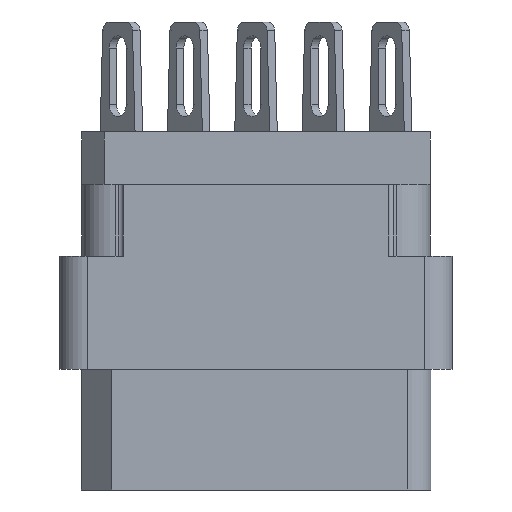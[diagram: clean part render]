
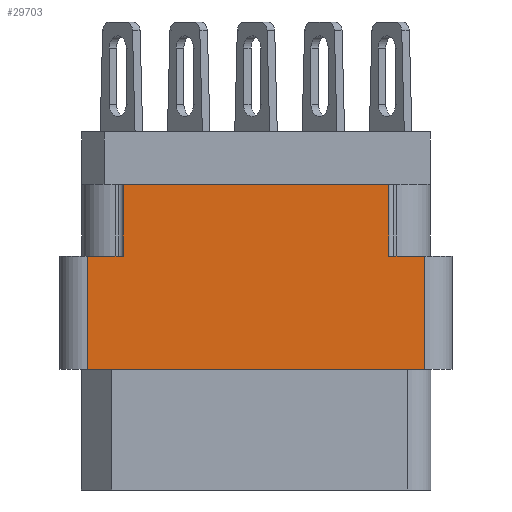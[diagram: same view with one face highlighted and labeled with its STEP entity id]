
A CAD part, left-side view. The second image highlights one B-rep face of the part: STEP entity #29703.
In plain terms, the highlighted planar face has unit normal (-1, 0, 0).
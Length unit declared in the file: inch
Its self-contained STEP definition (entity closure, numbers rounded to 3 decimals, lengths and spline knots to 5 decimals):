
#116 = CARTESIAN_POINT ( 'NONE',  ( -1., -0.376, -0.529 ) ) ;
#2129 = CARTESIAN_POINT ( 'NONE',  ( -1., -0.376, -0.529 ) ) ;
#2211 = LINE ( 'NONE', #35784, #32239 ) ;
#4123 = VECTOR ( 'NONE', #28141, 39.37008 ) ;
#4186 = ORIENTED_EDGE ( 'NONE', *, *, #26919, .F. ) ;
#4498 = DIRECTION ( 'NONE',  ( 0., -1., 0. ) ) ;
#4807 = DIRECTION ( 'NONE',  ( 0., -1., 0. ) ) ;
#5062 = CARTESIAN_POINT ( 'NONE',  ( -1., -0.296, -0.117 ) ) ;
#5085 = CARTESIAN_POINT ( 'NONE',  ( -1., -0.296, -0.277 ) ) ;
#5240 = LINE ( 'NONE', #19063, #13813 ) ;
#5653 = CARTESIAN_POINT ( 'NONE',  ( -1., 0.376, -0.798 ) ) ;
#5930 = VERTEX_POINT ( 'NONE', #9244 ) ;
#6096 = EDGE_CURVE ( 'NONE', #18663, #5930, #2211, .T. ) ;
#7786 = CARTESIAN_POINT ( 'NONE',  ( -1., 0.376, -0.529 ) ) ;
#9244 = CARTESIAN_POINT ( 'NONE',  ( -1., 0.296, -0.277 ) ) ;
#9344 = DIRECTION ( 'NONE',  ( -1., 0., 0. ) ) ;
#9796 = CARTESIAN_POINT ( 'NONE',  ( -1., -0.376, -0.277 ) ) ;
#10164 = VECTOR ( 'NONE', #32843, 39.37008 ) ;
#10178 = DIRECTION ( 'NONE',  ( 0., 0., 1. ) ) ;
#10691 = VERTEX_POINT ( 'NONE', #116 ) ;
#11288 = VECTOR ( 'NONE', #33193, 39.37008 ) ;
#11901 = EDGE_LOOP ( 'NONE', ( #26837, #4186, #26908, #22392, #35213, #28728, #31324, #19036 ) ) ;
#13813 = VECTOR ( 'NONE', #4498, 39.37008 ) ;
#13922 = DIRECTION ( 'NONE',  ( 0., 0., 1. ) ) ;
#14253 = VERTEX_POINT ( 'NONE', #9796 ) ;
#14954 = VERTEX_POINT ( 'NONE', #5062 ) ;
#15341 = EDGE_CURVE ( 'NONE', #10691, #14253, #30640, .T. ) ;
#15355 = VECTOR ( 'NONE', #18925, 39.37008 ) ;
#16679 = LINE ( 'NONE', #5085, #28107 ) ;
#18567 = FACE_OUTER_BOUND ( 'NONE', #11901, .T. ) ;
#18663 = VERTEX_POINT ( 'NONE', #21725 ) ;
#18925 = DIRECTION ( 'NONE',  ( 0., 1., 0. ) ) ;
#19036 = ORIENTED_EDGE ( 'NONE', *, *, #6096, .F. ) ;
#19063 = CARTESIAN_POINT ( 'NONE',  ( -1., 0.438, -0.117 ) ) ;
#19352 = VECTOR ( 'NONE', #10178, 39.37008 ) ;
#19531 = EDGE_CURVE ( 'NONE', #5930, #21313, #21591, .T. ) ;
#20542 = CARTESIAN_POINT ( 'NONE',  ( -1., -0.296, -0.277 ) ) ;
#21313 = VERTEX_POINT ( 'NONE', #34097 ) ;
#21591 = LINE ( 'NONE', #27662, #10164 ) ;
#21687 = LINE ( 'NONE', #2129, #15355 ) ;
#21725 = CARTESIAN_POINT ( 'NONE',  ( -1., 0.376, -0.277 ) ) ;
#22021 = AXIS2_PLACEMENT_3D ( 'NONE', #29068, #9344, #29811 ) ;
#22392 = ORIENTED_EDGE ( 'NONE', *, *, #25352, .F. ) ;
#24556 = CARTESIAN_POINT ( 'NONE',  ( -1., -0.376, -0.798 ) ) ;
#24701 = EDGE_CURVE ( 'NONE', #31984, #18663, #27955, .T. ) ;
#25352 = EDGE_CURVE ( 'NONE', #27173, #14253, #27096, .T. ) ;
#26837 = ORIENTED_EDGE ( 'NONE', *, *, #24701, .F. ) ;
#26908 = ORIENTED_EDGE ( 'NONE', *, *, #15341, .T. ) ;
#26919 = EDGE_CURVE ( 'NONE', #10691, #31984, #21687, .T. ) ;
#27096 = LINE ( 'NONE', #33383, #11288 ) ;
#27173 = VERTEX_POINT ( 'NONE', #20542 ) ;
#27662 = CARTESIAN_POINT ( 'NONE',  ( -1., 0.296, -0.277 ) ) ;
#27955 = LINE ( 'NONE', #5653, #4123 ) ;
#28107 = VECTOR ( 'NONE', #13922, 39.37008 ) ;
#28141 = DIRECTION ( 'NONE',  ( 0., 0., 1. ) ) ;
#28728 = ORIENTED_EDGE ( 'NONE', *, *, #30342, .F. ) ;
#29068 = CARTESIAN_POINT ( 'NONE',  ( -1., -0.376, -0.798 ) ) ;
#29703 = ADVANCED_FACE ( 'NONE', ( #18567 ), #34600, .T. ) ;
#29811 = DIRECTION ( 'NONE',  ( 0., 0., 1. ) ) ;
#30342 = EDGE_CURVE ( 'NONE', #21313, #14954, #5240, .T. ) ;
#30640 = LINE ( 'NONE', #24556, #19352 ) ;
#31324 = ORIENTED_EDGE ( 'NONE', *, *, #19531, .F. ) ;
#31984 = VERTEX_POINT ( 'NONE', #7786 ) ;
#32239 = VECTOR ( 'NONE', #4807, 39.37008 ) ;
#32843 = DIRECTION ( 'NONE',  ( 0., 0., 1. ) ) ;
#33193 = DIRECTION ( 'NONE',  ( 0., -1., 0. ) ) ;
#33383 = CARTESIAN_POINT ( 'NONE',  ( -1., -0.296, -0.277 ) ) ;
#33547 = EDGE_CURVE ( 'NONE', #27173, #14954, #16679, .T. ) ;
#34097 = CARTESIAN_POINT ( 'NONE',  ( -1., 0.296, -0.117 ) ) ;
#34600 = PLANE ( 'NONE',  #22021 ) ;
#35213 = ORIENTED_EDGE ( 'NONE', *, *, #33547, .T. ) ;
#35784 = CARTESIAN_POINT ( 'NONE',  ( -1., 0.438, -0.277 ) ) ;
